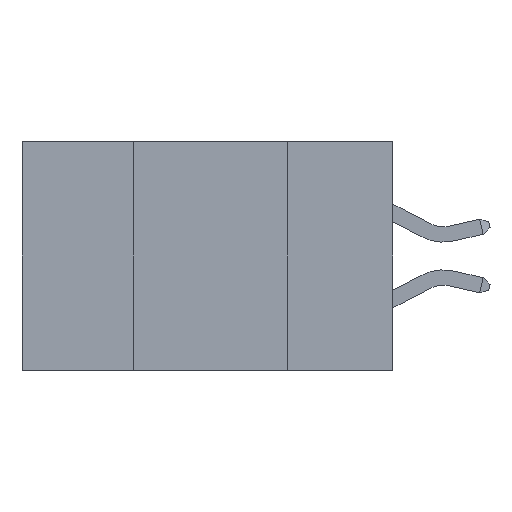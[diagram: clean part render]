
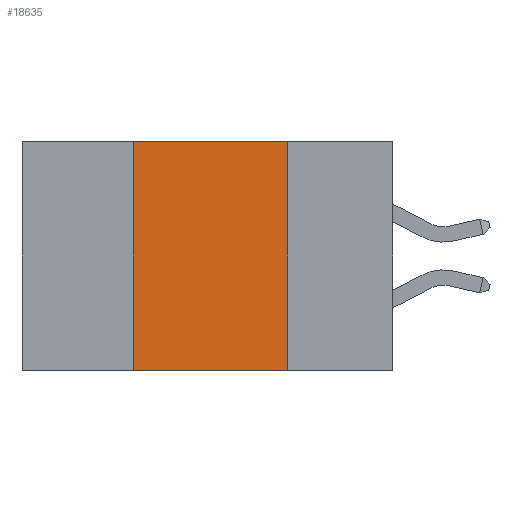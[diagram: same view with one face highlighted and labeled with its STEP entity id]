
A CAD part, left-side view. The second image highlights one B-rep face of the part: STEP entity #18635.
In plain terms, the highlighted planar face has unit normal (-1, 0, 0).
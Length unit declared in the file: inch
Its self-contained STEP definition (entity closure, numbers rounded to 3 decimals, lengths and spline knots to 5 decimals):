
#722 = EDGE_CURVE ( 'NONE', #7969, #5171, #5954, .T. ) ;
#2767 = AXIS2_PLACEMENT_3D ( 'NONE', #23585, #3023, #17549 ) ;
#3008 = CARTESIAN_POINT ( 'NONE',  ( 0., 0.17, -0.37 ) ) ;
#3023 = DIRECTION ( 'NONE',  ( 1., 0., 0. ) ) ;
#3437 = CARTESIAN_POINT ( 'NONE',  ( 0., 0.42, -0.37 ) ) ;
#4759 = FACE_OUTER_BOUND ( 'NONE', #9262, .T. ) ;
#4936 = CARTESIAN_POINT ( 'NONE',  ( 0., 0.17, 0. ) ) ;
#5171 = VERTEX_POINT ( 'NONE', #12107 ) ;
#5342 = ORIENTED_EDGE ( 'NONE', *, *, #722, .F. ) ;
#5557 = VERTEX_POINT ( 'NONE', #3008 ) ;
#5639 = VECTOR ( 'NONE', #22019, 39.37008 ) ;
#5954 = LINE ( 'NONE', #13776, #6610 ) ;
#6610 = VECTOR ( 'NONE', #25901, 39.37008 ) ;
#6890 = VECTOR ( 'NONE', #25455, 39.37008 ) ;
#7106 = EDGE_CURVE ( 'NONE', #18077, #5557, #20311, .T. ) ;
#7547 = LINE ( 'NONE', #4936, #6890 ) ;
#7969 = VERTEX_POINT ( 'NONE', #24574 ) ;
#9262 = EDGE_LOOP ( 'NONE', ( #12873, #5342, #14795, #18085 ) ) ;
#12107 = CARTESIAN_POINT ( 'NONE',  ( 0., 0.17, 0. ) ) ;
#12873 = ORIENTED_EDGE ( 'NONE', *, *, #26614, .F. ) ;
#13776 = CARTESIAN_POINT ( 'NONE',  ( 0., 0.6, 0. ) ) ;
#14795 = ORIENTED_EDGE ( 'NONE', *, *, #19545, .F. ) ;
#14884 = VECTOR ( 'NONE', #15859, 39.37008 ) ;
#15859 = DIRECTION ( 'NONE',  ( 0., -1., 0. ) ) ;
#17549 = DIRECTION ( 'NONE',  ( 0., 0., -1. ) ) ;
#17915 = CARTESIAN_POINT ( 'NONE',  ( 0., 0.42, 0. ) ) ;
#18077 = VERTEX_POINT ( 'NONE', #3437 ) ;
#18085 = ORIENTED_EDGE ( 'NONE', *, *, #7106, .T. ) ;
#18635 = ADVANCED_FACE ( 'NONE', ( #4759 ), #25594, .F. ) ;
#19545 = EDGE_CURVE ( 'NONE', #18077, #7969, #22081, .T. ) ;
#19863 = CARTESIAN_POINT ( 'NONE',  ( 0., 0.6, -0.37 ) ) ;
#20311 = LINE ( 'NONE', #19863, #14884 ) ;
#22019 = DIRECTION ( 'NONE',  ( 0., 0., 1. ) ) ;
#22081 = LINE ( 'NONE', #17915, #5639 ) ;
#23585 = CARTESIAN_POINT ( 'NONE',  ( 0., 0.6, 0. ) ) ;
#24574 = CARTESIAN_POINT ( 'NONE',  ( 0., 0.42, 0. ) ) ;
#25455 = DIRECTION ( 'NONE',  ( 0., 0., -1. ) ) ;
#25594 = PLANE ( 'NONE',  #2767 ) ;
#25901 = DIRECTION ( 'NONE',  ( 0., -1., 0. ) ) ;
#26614 = EDGE_CURVE ( 'NONE', #5171, #5557, #7547, .T. ) ;
